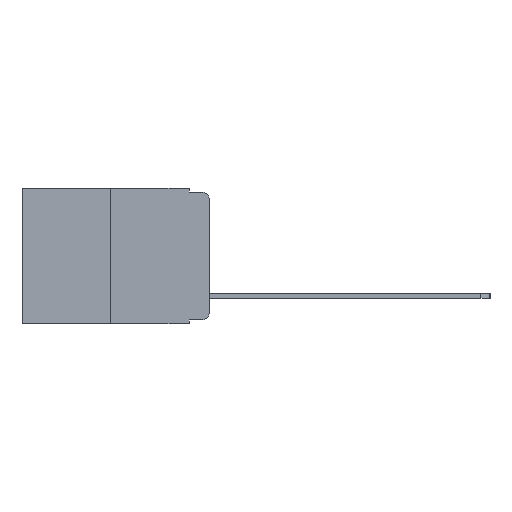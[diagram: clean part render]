
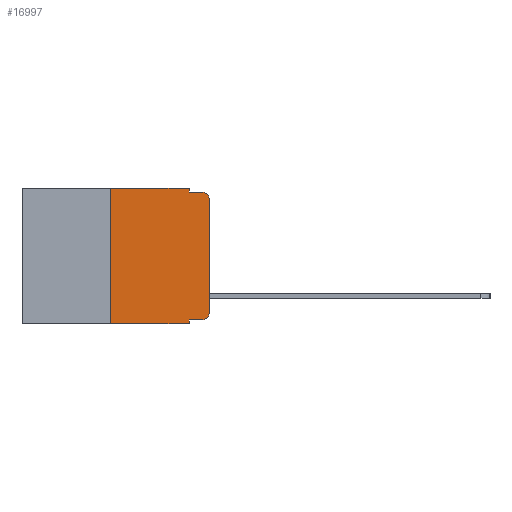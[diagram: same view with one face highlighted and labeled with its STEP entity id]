
A CAD part, left-side view. The second image highlights one B-rep face of the part: STEP entity #16997.
In plain terms, the highlighted planar face has unit normal (-1, 0, 0).
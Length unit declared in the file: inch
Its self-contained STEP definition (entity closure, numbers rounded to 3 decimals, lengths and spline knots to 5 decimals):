
#45 = VERTEX_POINT ( 'NONE', #127 ) ;
#127 = CARTESIAN_POINT ( 'NONE',  ( 0., 0.25, 0. ) ) ;
#435 = ORIENTED_EDGE ( 'NONE', *, *, #1413, .T. ) ;
#476 = VERTEX_POINT ( 'NONE', #5217 ) ;
#693 = LINE ( 'NONE', #10608, #8751 ) ;
#711 = CARTESIAN_POINT ( 'NONE',  ( 0., 0.02, -0.03 ) ) ;
#1269 = EDGE_CURVE ( 'NONE', #6395, #3287, #7367, .T. ) ;
#1413 = EDGE_CURVE ( 'NONE', #15839, #9029, #18512, .T. ) ;
#1580 = DIRECTION ( 'NONE',  ( -1., 0., 0. ) ) ;
#1613 = CARTESIAN_POINT ( 'NONE',  ( 0., 0.25, 0. ) ) ;
#1637 = DIRECTION ( 'NONE',  ( 0., 0., -1. ) ) ;
#1678 = DIRECTION ( 'NONE',  ( 0., 0., 1. ) ) ;
#1819 = CARTESIAN_POINT ( 'NONE',  ( 0., 0., -0.03 ) ) ;
#1870 = ORIENTED_EDGE ( 'NONE', *, *, #4103, .T. ) ;
#2351 = EDGE_CURVE ( 'NONE', #476, #9029, #14291, .T. ) ;
#2510 = VECTOR ( 'NONE', #12313, 39.37008 ) ;
#2751 = LINE ( 'NONE', #11775, #9758 ) ;
#2867 = FACE_OUTER_BOUND ( 'NONE', #11249, .T. ) ;
#3040 = CARTESIAN_POINT ( 'NONE',  ( 0., 0.02, -0.313 ) ) ;
#3287 = VERTEX_POINT ( 'NONE', #6690 ) ;
#3317 = VECTOR ( 'NONE', #4570, 39.37008 ) ;
#3517 = LINE ( 'NONE', #1613, #18076 ) ;
#3820 = ORIENTED_EDGE ( 'NONE', *, *, #1269, .T. ) ;
#3843 = EDGE_CURVE ( 'NONE', #4029, #9537, #18050, .T. ) ;
#3995 = CARTESIAN_POINT ( 'NONE',  ( 0., 0.02, -0.01 ) ) ;
#4029 = VERTEX_POINT ( 'NONE', #17053 ) ;
#4103 = EDGE_CURVE ( 'NONE', #6666, #15839, #2751, .T. ) ;
#4177 = CARTESIAN_POINT ( 'NONE',  ( 0., 0.02, -0.333 ) ) ;
#4289 = LINE ( 'NONE', #7234, #15175 ) ;
#4570 = DIRECTION ( 'NONE',  ( 0., -1., 0. ) ) ;
#4587 = DIRECTION ( 'NONE',  ( 0., 0., -1. ) ) ;
#4794 = EDGE_CURVE ( 'NONE', #9537, #6666, #8133, .T. ) ;
#5196 = CARTESIAN_POINT ( 'NONE',  ( 0., 0.051, -0.333 ) ) ;
#5217 = CARTESIAN_POINT ( 'NONE',  ( 0., 0.051, -0.01 ) ) ;
#6318 = CARTESIAN_POINT ( 'NONE',  ( 0., 0.473, 0. ) ) ;
#6395 = VERTEX_POINT ( 'NONE', #8633 ) ;
#6428 = VECTOR ( 'NONE', #17227, 39.37008 ) ;
#6666 = VERTEX_POINT ( 'NONE', #10945 ) ;
#6690 = CARTESIAN_POINT ( 'NONE',  ( 0., 0.051, -0.343 ) ) ;
#6695 = AXIS2_PLACEMENT_3D ( 'NONE', #6318, #16038, #7759 ) ;
#6896 = EDGE_CURVE ( 'NONE', #4029, #3287, #8933, .T. ) ;
#7056 = AXIS2_PLACEMENT_3D ( 'NONE', #711, #1580, #1637 ) ;
#7234 = CARTESIAN_POINT ( 'NONE',  ( 0., 0.473, 0. ) ) ;
#7241 = CARTESIAN_POINT ( 'NONE',  ( 0., 0.051, 0. ) ) ;
#7367 = LINE ( 'NONE', #11554, #3317 ) ;
#7666 = EDGE_CURVE ( 'NONE', #6395, #45, #3517, .T. ) ;
#7759 = DIRECTION ( 'NONE',  ( 0., 0., -1. ) ) ;
#8133 = CIRCLE ( 'NONE', #17087, 0.02 ) ;
#8534 = ORIENTED_EDGE ( 'NONE', *, *, #4794, .T. ) ;
#8633 = CARTESIAN_POINT ( 'NONE',  ( 0., 0.25, -0.343 ) ) ;
#8751 = VECTOR ( 'NONE', #17390, 39.37008 ) ;
#8933 = LINE ( 'NONE', #7241, #11315 ) ;
#9029 = VERTEX_POINT ( 'NONE', #3995 ) ;
#9168 = PLANE ( 'NONE',  #6695 ) ;
#9537 = VERTEX_POINT ( 'NONE', #4177 ) ;
#9639 = ORIENTED_EDGE ( 'NONE', *, *, #7666, .F. ) ;
#9758 = VECTOR ( 'NONE', #13150, 39.37008 ) ;
#10608 = CARTESIAN_POINT ( 'NONE',  ( 0., 0.051, 0. ) ) ;
#10945 = CARTESIAN_POINT ( 'NONE',  ( 0., 0., -0.313 ) ) ;
#11249 = EDGE_LOOP ( 'NONE', ( #1870, #435, #15398, #17297, #13705, #9639, #3820, #13509, #13081, #8534 ) ) ;
#11315 = VECTOR ( 'NONE', #16994, 39.37008 ) ;
#11554 = CARTESIAN_POINT ( 'NONE',  ( 0., 0.473, -0.343 ) ) ;
#11775 = CARTESIAN_POINT ( 'NONE',  ( 0., 0., 0. ) ) ;
#12239 = EDGE_CURVE ( 'NONE', #45, #13117, #4289, .T. ) ;
#12313 = DIRECTION ( 'NONE',  ( 0., -1., 0. ) ) ;
#12844 = DIRECTION ( 'NONE',  ( 0., -1., 0. ) ) ;
#13081 = ORIENTED_EDGE ( 'NONE', *, *, #3843, .T. ) ;
#13117 = VERTEX_POINT ( 'NONE', #17466 ) ;
#13150 = DIRECTION ( 'NONE',  ( 0., 0., 1. ) ) ;
#13166 = DIRECTION ( 'NONE',  ( -1., 0., 0. ) ) ;
#13509 = ORIENTED_EDGE ( 'NONE', *, *, #6896, .F. ) ;
#13705 = ORIENTED_EDGE ( 'NONE', *, *, #12239, .F. ) ;
#14291 = LINE ( 'NONE', #16654, #6428 ) ;
#15175 = VECTOR ( 'NONE', #12844, 39.37008 ) ;
#15398 = ORIENTED_EDGE ( 'NONE', *, *, #2351, .F. ) ;
#15839 = VERTEX_POINT ( 'NONE', #1819 ) ;
#16038 = DIRECTION ( 'NONE',  ( 1., 0., 0. ) ) ;
#16654 = CARTESIAN_POINT ( 'NONE',  ( 0., 0.051, -0.01 ) ) ;
#16994 = DIRECTION ( 'NONE',  ( 0., 0., -1. ) ) ;
#16997 = ADVANCED_FACE ( 'NONE', ( #2867 ), #9168, .F. ) ;
#17053 = CARTESIAN_POINT ( 'NONE',  ( 0., 0.051, -0.333 ) ) ;
#17087 = AXIS2_PLACEMENT_3D ( 'NONE', #3040, #13166, #4587 ) ;
#17227 = DIRECTION ( 'NONE',  ( 0., -1., 0. ) ) ;
#17297 = ORIENTED_EDGE ( 'NONE', *, *, #18521, .F. ) ;
#17390 = DIRECTION ( 'NONE',  ( 0., 0., -1. ) ) ;
#17466 = CARTESIAN_POINT ( 'NONE',  ( 0., 0.051, 0. ) ) ;
#18050 = LINE ( 'NONE', #5196, #2510 ) ;
#18076 = VECTOR ( 'NONE', #1678, 39.37008 ) ;
#18512 = CIRCLE ( 'NONE', #7056, 0.02 ) ;
#18521 = EDGE_CURVE ( 'NONE', #13117, #476, #693, .T. ) ;
